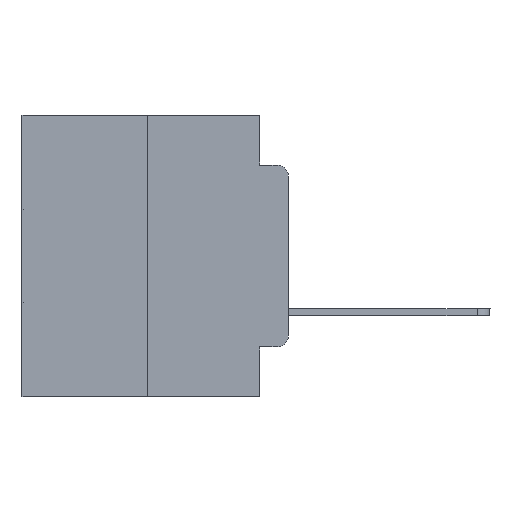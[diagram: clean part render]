
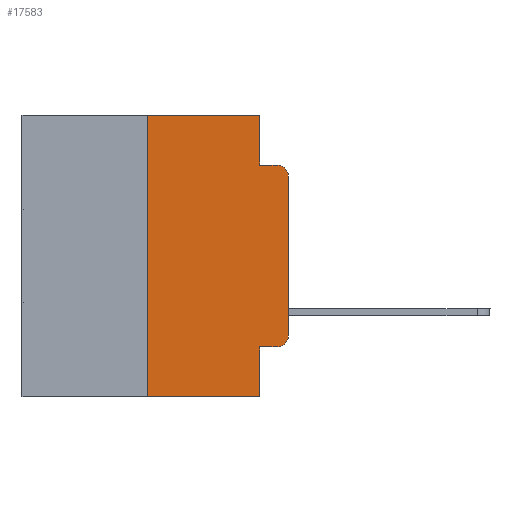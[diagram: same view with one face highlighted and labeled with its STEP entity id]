
A CAD part, left-side view. The second image highlights one B-rep face of the part: STEP entity #17583.
In plain terms, the highlighted planar face has unit normal (-1, 0, 0).
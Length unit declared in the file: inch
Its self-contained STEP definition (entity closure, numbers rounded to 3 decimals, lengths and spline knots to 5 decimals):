
#52 = DIRECTION ( 'NONE',  ( 0., 0., 1. ) ) ;
#262 = VECTOR ( 'NONE', #4879, 39.37008 ) ;
#379 = VECTOR ( 'NONE', #19472, 39.37008 ) ;
#1179 = ORIENTED_EDGE ( 'NONE', *, *, #3961, .F. ) ;
#1394 = EDGE_CURVE ( 'NONE', #7815, #19622, #4656, .T. ) ;
#1439 = VERTEX_POINT ( 'NONE', #7974 ) ;
#1456 = DIRECTION ( 'NONE',  ( -1., 0., 0. ) ) ;
#1704 = CARTESIAN_POINT ( 'NONE',  ( 0., 0.051, 0. ) ) ;
#2451 = VECTOR ( 'NONE', #14658, 39.37008 ) ;
#2547 = ORIENTED_EDGE ( 'NONE', *, *, #26479, .F. ) ;
#2922 = FACE_OUTER_BOUND ( 'NONE', #27027, .T. ) ;
#3355 = VECTOR ( 'NONE', #52, 39.37008 ) ;
#3961 = EDGE_CURVE ( 'NONE', #23837, #20992, #7220, .T. ) ;
#4323 = AXIS2_PLACEMENT_3D ( 'NONE', #23193, #27478, #22999 ) ;
#4656 = CIRCLE ( 'NONE', #4323, 0.02 ) ;
#4879 = DIRECTION ( 'NONE',  ( 0., -1., 0. ) ) ;
#5520 = DIRECTION ( 'NONE',  ( 0., -1., 0. ) ) ;
#5806 = CARTESIAN_POINT ( 'NONE',  ( 0., 0.25, -0.5 ) ) ;
#7220 = LINE ( 'NONE', #12432, #24015 ) ;
#7815 = VERTEX_POINT ( 'NONE', #25877 ) ;
#7974 = CARTESIAN_POINT ( 'NONE',  ( 0., 0.051, -0.5 ) ) ;
#8272 = LINE ( 'NONE', #1704, #2451 ) ;
#8573 = EDGE_CURVE ( 'NONE', #22028, #7815, #13615, .T. ) ;
#8948 = ORIENTED_EDGE ( 'NONE', *, *, #24644, .F. ) ;
#9780 = VECTOR ( 'NONE', #28246, 39.37008 ) ;
#9817 = CARTESIAN_POINT ( 'NONE',  ( 0., 0.02, -0.4115 ) ) ;
#9944 = CARTESIAN_POINT ( 'NONE',  ( 0., 0., -0.3915 ) ) ;
#10314 = LINE ( 'NONE', #15111, #379 ) ;
#10332 = EDGE_CURVE ( 'NONE', #23899, #18268, #23474, .T. ) ;
#11283 = CARTESIAN_POINT ( 'NONE',  ( 0., 0.473, 0. ) ) ;
#11359 = EDGE_CURVE ( 'NONE', #23837, #1439, #27143, .T. ) ;
#12207 = ORIENTED_EDGE ( 'NONE', *, *, #8573, .T. ) ;
#12432 = CARTESIAN_POINT ( 'NONE',  ( 0., 0.25, 0. ) ) ;
#12769 = CARTESIAN_POINT ( 'NONE',  ( 0., 0.02, -0.0885 ) ) ;
#12920 = CARTESIAN_POINT ( 'NONE',  ( 0., 0.051, -0.4115 ) ) ;
#13228 = EDGE_CURVE ( 'NONE', #19279, #19622, #10314, .T. ) ;
#13424 = CARTESIAN_POINT ( 'NONE',  ( 0., 0.051, 0. ) ) ;
#13615 = LINE ( 'NONE', #15070, #3355 ) ;
#14658 = DIRECTION ( 'NONE',  ( 0., 0., -1. ) ) ;
#14894 = CARTESIAN_POINT ( 'NONE',  ( 0., 0.25, 0. ) ) ;
#15070 = CARTESIAN_POINT ( 'NONE',  ( 0., 0., 0. ) ) ;
#15111 = CARTESIAN_POINT ( 'NONE',  ( 0., 0.051, -0.0885 ) ) ;
#15595 = DIRECTION ( 'NONE',  ( 1., 0., 0. ) ) ;
#15656 = EDGE_CURVE ( 'NONE', #18268, #22028, #19143, .T. ) ;
#15880 = CARTESIAN_POINT ( 'NONE',  ( 0., 0.473, 0. ) ) ;
#16448 = ORIENTED_EDGE ( 'NONE', *, *, #13228, .F. ) ;
#16559 = CARTESIAN_POINT ( 'NONE',  ( 0., 0.051, -0.4115 ) ) ;
#16674 = ORIENTED_EDGE ( 'NONE', *, *, #23534, .F. ) ;
#16709 = DIRECTION ( 'NONE',  ( 0., 0., -1. ) ) ;
#16727 = AXIS2_PLACEMENT_3D ( 'NONE', #11283, #15595, #26547 ) ;
#16807 = CARTESIAN_POINT ( 'NONE',  ( 0., 0.02, -0.3915 ) ) ;
#16949 = VERTEX_POINT ( 'NONE', #13424 ) ;
#17583 = ADVANCED_FACE ( 'NONE', ( #2922 ), #19875, .F. ) ;
#17992 = ORIENTED_EDGE ( 'NONE', *, *, #11359, .T. ) ;
#18268 = VERTEX_POINT ( 'NONE', #9817 ) ;
#18550 = ORIENTED_EDGE ( 'NONE', *, *, #10332, .T. ) ;
#18926 = VECTOR ( 'NONE', #19125, 39.37008 ) ;
#19125 = DIRECTION ( 'NONE',  ( 0., -1., 0. ) ) ;
#19143 = CIRCLE ( 'NONE', #24386, 0.02 ) ;
#19203 = DIRECTION ( 'NONE',  ( 0., 0., 1. ) ) ;
#19279 = VERTEX_POINT ( 'NONE', #24105 ) ;
#19472 = DIRECTION ( 'NONE',  ( 0., -1., 0. ) ) ;
#19622 = VERTEX_POINT ( 'NONE', #12769 ) ;
#19875 = PLANE ( 'NONE',  #16727 ) ;
#20992 = VERTEX_POINT ( 'NONE', #14894 ) ;
#22028 = VERTEX_POINT ( 'NONE', #9944 ) ;
#22082 = LINE ( 'NONE', #28150, #9780 ) ;
#22764 = ORIENTED_EDGE ( 'NONE', *, *, #15656, .T. ) ;
#22999 = DIRECTION ( 'NONE',  ( 0., 0., -1. ) ) ;
#23193 = CARTESIAN_POINT ( 'NONE',  ( 0., 0.02, -0.1085 ) ) ;
#23474 = LINE ( 'NONE', #16559, #25849 ) ;
#23534 = EDGE_CURVE ( 'NONE', #20992, #16949, #27608, .T. ) ;
#23837 = VERTEX_POINT ( 'NONE', #5806 ) ;
#23899 = VERTEX_POINT ( 'NONE', #12920 ) ;
#24015 = VECTOR ( 'NONE', #19203, 39.37008 ) ;
#24105 = CARTESIAN_POINT ( 'NONE',  ( 0., 0.051, -0.0885 ) ) ;
#24386 = AXIS2_PLACEMENT_3D ( 'NONE', #16807, #1456, #16709 ) ;
#24644 = EDGE_CURVE ( 'NONE', #23899, #1439, #22082, .T. ) ;
#25849 = VECTOR ( 'NONE', #5520, 39.37008 ) ;
#25877 = CARTESIAN_POINT ( 'NONE',  ( 0., 0., -0.1085 ) ) ;
#26479 = EDGE_CURVE ( 'NONE', #16949, #19279, #8272, .T. ) ;
#26547 = DIRECTION ( 'NONE',  ( 0., 0., -1. ) ) ;
#27027 = EDGE_LOOP ( 'NONE', ( #12207, #27113, #16448, #2547, #16674, #1179, #17992, #8948, #18550, #22764 ) ) ;
#27113 = ORIENTED_EDGE ( 'NONE', *, *, #1394, .T. ) ;
#27143 = LINE ( 'NONE', #27819, #18926 ) ;
#27478 = DIRECTION ( 'NONE',  ( -1., 0., 0. ) ) ;
#27608 = LINE ( 'NONE', #15880, #262 ) ;
#27819 = CARTESIAN_POINT ( 'NONE',  ( 0., 0.473, -0.5 ) ) ;
#28150 = CARTESIAN_POINT ( 'NONE',  ( 0., 0.051, 0. ) ) ;
#28246 = DIRECTION ( 'NONE',  ( 0., 0., -1. ) ) ;
